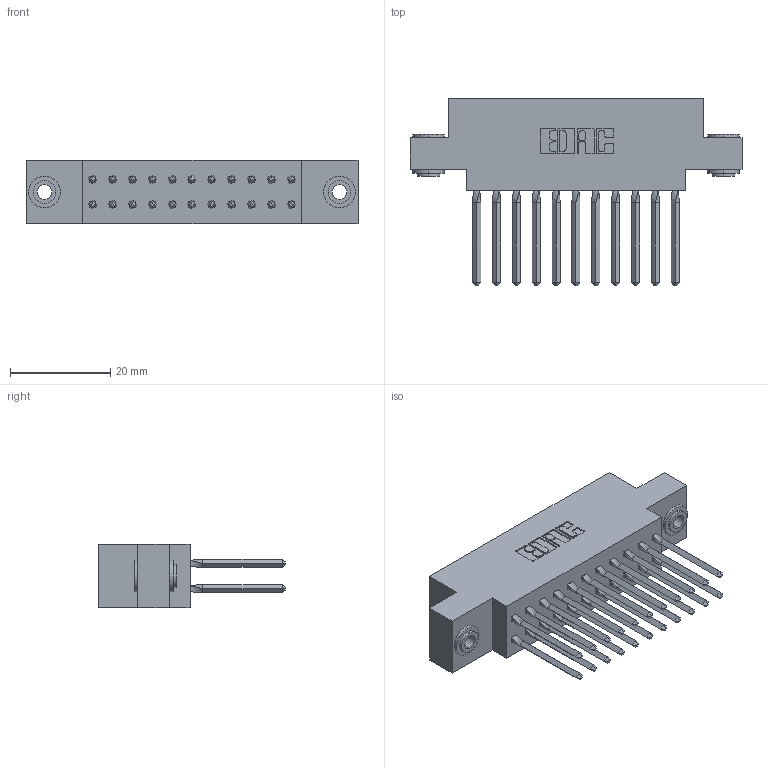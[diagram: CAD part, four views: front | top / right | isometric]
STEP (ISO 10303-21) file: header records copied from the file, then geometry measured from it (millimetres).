
FILE_DESCRIPTION (( 'STEP AP203' ), '1' );
FILE_NAME ('317-022-540-803.STEP', '2020-02-27T17:22:20', ( '' ), ( '' ), 'SwSTEP 2.0', 'SolidWorks 2016', '' );
FILE_SCHEMA (( 'CONFIG_CONTROL_DESIGN' ));
Length unit declared in the file: inch
Products named in the file (4): 345-250-002_345-250-002-102; 317 Part_.156 Dia - TH; 317-290-001_540; 317-022-540-803
Assembly tree (25 placements, depth 2):
  317-022-540-803
    317 Part_.156 Dia - TH
    317-290-001_540  x22
    345-250-002_345-250-002-102  x2
Bounding box: 66.29 x 37.34 x 12.7 mm (x, y, z)
Volume: 10097.4 mm3; surface area: 14096.7 mm2
Topology: 25 solids, 25 shells, 2098 faces, 5785 edges, 3728 vertices
Faces by surface type: plane 1674, cylinder 328, bspline 88, cone 8
Entity records: 20875 total; most frequent: CARTESIAN_POINT 4022, ORIENTED_EDGE 3514, DIRECTION 2977, EDGE_CURVE 1757, LINE 1477, VECTOR 1477, VERTEX_POINT 1163, AXIS2_PLACEMENT_3D 750
